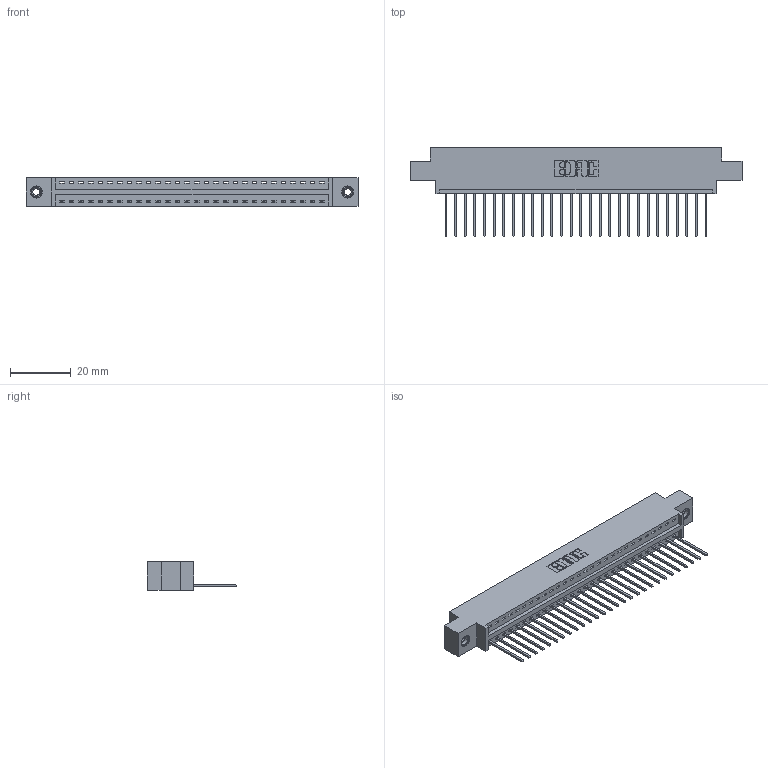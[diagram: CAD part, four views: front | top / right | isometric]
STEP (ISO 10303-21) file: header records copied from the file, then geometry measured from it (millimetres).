
FILE_DESCRIPTION (( 'STEP AP203' ), '1' );
FILE_NAME ('396-028-540-608.STEP', '2019-10-27T08:57:44', ( '' ), ( '' ), 'SwSTEP 2.0', 'SolidWorks 2016', '' );
FILE_SCHEMA (( 'CONFIG_CONTROL_DESIGN' ));
Length unit declared in the file: inch
Products named in the file (4): 345-292-001_345-293-140; 345-250-001_345-250-003-102; 346 Part_0.170 Offset - 0.156 Dia-TI; 396-028-540-608
Assembly tree (31 placements, depth 2):
  396-028-540-608
    346 Part_0.170 Offset - 0.156 Dia-TI
    345-292-001_345-293-140  x28
    345-250-001_345-250-003-102  x2
Bounding box: 109.47 x 29.46 x 9.4 mm (x, y, z)
Volume: 10259.4 mm3; surface area: 13130.8 mm2
Topology: 31 solids, 31 shells, 1810 faces, 5405 edges, 3558 vertices
Faces by surface type: plane 1232, cylinder 562, cone 12, torus 4
Entity records: 20598 total; most frequent: CARTESIAN_POINT 3519, ORIENTED_EDGE 3474, DIRECTION 3147, EDGE_CURVE 1737, LINE 1473, VECTOR 1473, VERTEX_POINT 1152, AXIS2_PLACEMENT_3D 837
